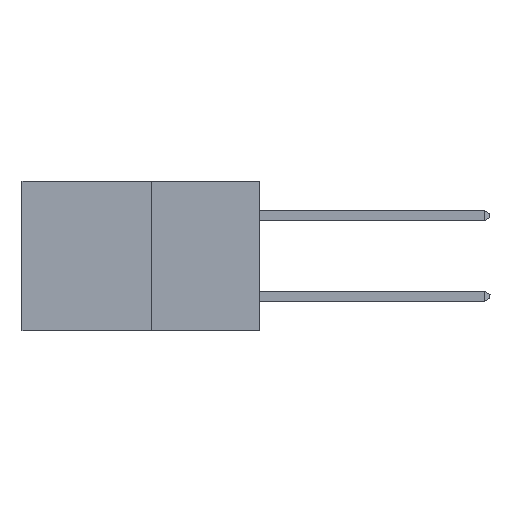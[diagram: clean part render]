
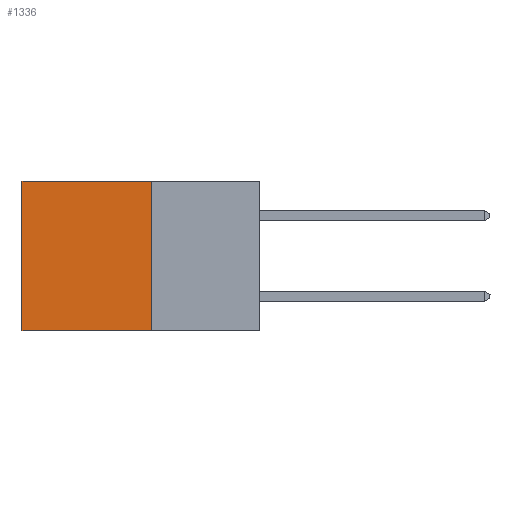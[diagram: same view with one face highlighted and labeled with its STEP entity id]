
A CAD part, left-side view. The second image highlights one B-rep face of the part: STEP entity #1336.
In plain terms, the highlighted planar face has unit normal (-1, 0, 0).
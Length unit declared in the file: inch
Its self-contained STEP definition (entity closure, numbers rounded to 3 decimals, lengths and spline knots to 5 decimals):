
#173 = EDGE_LOOP ( 'NONE', ( #658, #4041, #9038, #8033 ) ) ;
#291 = DIRECTION ( 'NONE',  ( 0., 0., -1. ) ) ;
#658 = ORIENTED_EDGE ( 'NONE', *, *, #5149, .T. ) ;
#732 = EDGE_CURVE ( 'NONE', #1679, #4266, #6524, .T. ) ;
#1049 = VERTEX_POINT ( 'NONE', #2657 ) ;
#1336 = ADVANCED_FACE ( 'NONE', ( #7522 ), #9616, .F. ) ;
#1679 = VERTEX_POINT ( 'NONE', #2067 ) ;
#1826 = LINE ( 'NONE', #10110, #3261 ) ;
#2067 = CARTESIAN_POINT ( 'NONE',  ( 0.277, 0.27, 0. ) ) ;
#2074 = LINE ( 'NONE', #9997, #8161 ) ;
#2657 = CARTESIAN_POINT ( 'NONE',  ( 0.277, 0.27, -0.37 ) ) ;
#2844 = CARTESIAN_POINT ( 'NONE',  ( 0.277, 0.59, 0. ) ) ;
#3128 = EDGE_CURVE ( 'NONE', #1049, #4842, #10215, .T. ) ;
#3261 = VECTOR ( 'NONE', #291, 39.37008 ) ;
#4041 = ORIENTED_EDGE ( 'NONE', *, *, #3128, .F. ) ;
#4186 = VECTOR ( 'NONE', #4418, 39.37008 ) ;
#4266 = VERTEX_POINT ( 'NONE', #2844 ) ;
#4418 = DIRECTION ( 'NONE',  ( 0., 1., 0. ) ) ;
#4842 = VERTEX_POINT ( 'NONE', #5348 ) ;
#4950 = DIRECTION ( 'NONE',  ( 1., 0., 0. ) ) ;
#5149 = EDGE_CURVE ( 'NONE', #4266, #4842, #1826, .T. ) ;
#5348 = CARTESIAN_POINT ( 'NONE',  ( 0.277, 0.59, -0.37 ) ) ;
#5694 = CARTESIAN_POINT ( 'NONE',  ( 0.277, 0.27, -0.37 ) ) ;
#6502 = CARTESIAN_POINT ( 'NONE',  ( 0.277, 0.27, -0.37 ) ) ;
#6524 = LINE ( 'NONE', #9950, #8265 ) ;
#6652 = DIRECTION ( 'NONE',  ( 0., 0., -1. ) ) ;
#6945 = EDGE_CURVE ( 'NONE', #1679, #1049, #2074, .T. ) ;
#7257 = DIRECTION ( 'NONE',  ( 0., 1., 0. ) ) ;
#7522 = FACE_OUTER_BOUND ( 'NONE', #173, .T. ) ;
#8033 = ORIENTED_EDGE ( 'NONE', *, *, #732, .T. ) ;
#8161 = VECTOR ( 'NONE', #9933, 39.37008 ) ;
#8265 = VECTOR ( 'NONE', #7257, 39.37008 ) ;
#9038 = ORIENTED_EDGE ( 'NONE', *, *, #6945, .F. ) ;
#9616 = PLANE ( 'NONE',  #9927 ) ;
#9927 = AXIS2_PLACEMENT_3D ( 'NONE', #5694, #4950, #6652 ) ;
#9933 = DIRECTION ( 'NONE',  ( 0., 0., -1. ) ) ;
#9950 = CARTESIAN_POINT ( 'NONE',  ( 0.277, 0.27, 0. ) ) ;
#9997 = CARTESIAN_POINT ( 'NONE',  ( 0.277, 0.27, -0.37 ) ) ;
#10110 = CARTESIAN_POINT ( 'NONE',  ( 0.277, 0.59, -0.37 ) ) ;
#10215 = LINE ( 'NONE', #6502, #4186 ) ;
